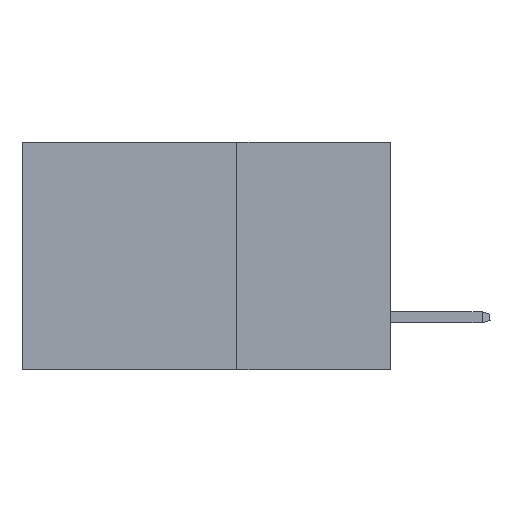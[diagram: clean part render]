
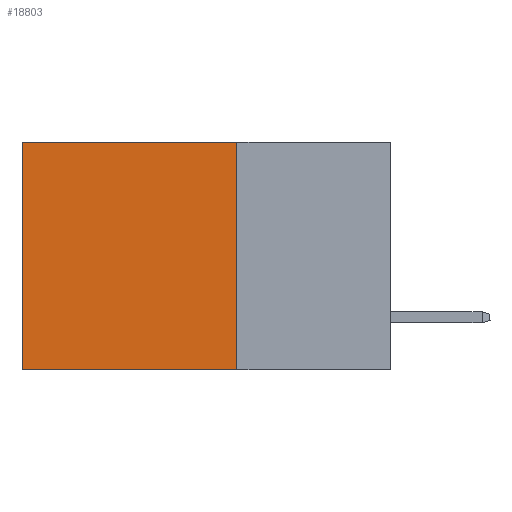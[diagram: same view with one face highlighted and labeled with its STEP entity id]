
A CAD part, left-side view. The second image highlights one B-rep face of the part: STEP entity #18803.
In plain terms, the highlighted planar face has unit normal (-1, 0, 0).
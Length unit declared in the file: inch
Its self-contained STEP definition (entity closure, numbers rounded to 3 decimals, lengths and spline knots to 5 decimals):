
#440 = VECTOR ( 'NONE', #30894, 39.37008 ) ;
#870 = PLANE ( 'NONE',  #4415 ) ;
#1996 = LINE ( 'NONE', #40051, #37835 ) ;
#4142 = VECTOR ( 'NONE', #6676, 39.37008 ) ;
#4415 = AXIS2_PLACEMENT_3D ( 'NONE', #44537, #26446, #4675 ) ;
#4497 = EDGE_CURVE ( 'NONE', #44531, #44762, #34310, .T. ) ;
#4675 = DIRECTION ( 'NONE',  ( 0., 0., -1. ) ) ;
#5349 = ORIENTED_EDGE ( 'NONE', *, *, #4497, .T. ) ;
#6676 = DIRECTION ( 'NONE',  ( 0., 1., 0. ) ) ;
#7605 = FACE_OUTER_BOUND ( 'NONE', #30369, .T. ) ;
#7844 = LINE ( 'NONE', #27221, #440 ) ;
#8625 = CARTESIAN_POINT ( 'NONE',  ( 0.2875, 0.6, -0.37 ) ) ;
#8674 = VERTEX_POINT ( 'NONE', #11905 ) ;
#9274 = ORIENTED_EDGE ( 'NONE', *, *, #37266, .F. ) ;
#10256 = ORIENTED_EDGE ( 'NONE', *, *, #43690, .F. ) ;
#11905 = CARTESIAN_POINT ( 'NONE',  ( 0.2875, 0.25, -0.37 ) ) ;
#17880 = CARTESIAN_POINT ( 'NONE',  ( 0.2875, 0.25, 0. ) ) ;
#18803 = ADVANCED_FACE ( 'NONE', ( #7605 ), #870, .F. ) ;
#22633 = VERTEX_POINT ( 'NONE', #8625 ) ;
#23134 = CARTESIAN_POINT ( 'NONE',  ( 0.2875, 0.25, 0. ) ) ;
#24083 = VECTOR ( 'NONE', #25364, 39.37008 ) ;
#25133 = DIRECTION ( 'NONE',  ( 0., 1., 0. ) ) ;
#25364 = DIRECTION ( 'NONE',  ( 0., 0., -1. ) ) ;
#26446 = DIRECTION ( 'NONE',  ( 1., 0., 0. ) ) ;
#27221 = CARTESIAN_POINT ( 'NONE',  ( 0.2875, 0.6, 0. ) ) ;
#30369 = EDGE_LOOP ( 'NONE', ( #35315, #10256, #9274, #5349 ) ) ;
#30894 = DIRECTION ( 'NONE',  ( 0., 0., -1. ) ) ;
#32288 = CARTESIAN_POINT ( 'NONE',  ( 0.2875, 0.25, 0. ) ) ;
#32393 = CARTESIAN_POINT ( 'NONE',  ( 0.2875, 0.6, 0. ) ) ;
#34310 = LINE ( 'NONE', #32288, #4142 ) ;
#35227 = EDGE_CURVE ( 'NONE', #44762, #22633, #7844, .T. ) ;
#35315 = ORIENTED_EDGE ( 'NONE', *, *, #35227, .T. ) ;
#37266 = EDGE_CURVE ( 'NONE', #44531, #8674, #41140, .T. ) ;
#37835 = VECTOR ( 'NONE', #25133, 39.37008 ) ;
#40051 = CARTESIAN_POINT ( 'NONE',  ( 0.2875, 0.25, -0.37 ) ) ;
#41140 = LINE ( 'NONE', #17880, #24083 ) ;
#43690 = EDGE_CURVE ( 'NONE', #8674, #22633, #1996, .T. ) ;
#44531 = VERTEX_POINT ( 'NONE', #23134 ) ;
#44537 = CARTESIAN_POINT ( 'NONE',  ( 0.2875, 0.25, 0. ) ) ;
#44762 = VERTEX_POINT ( 'NONE', #32393 ) ;
